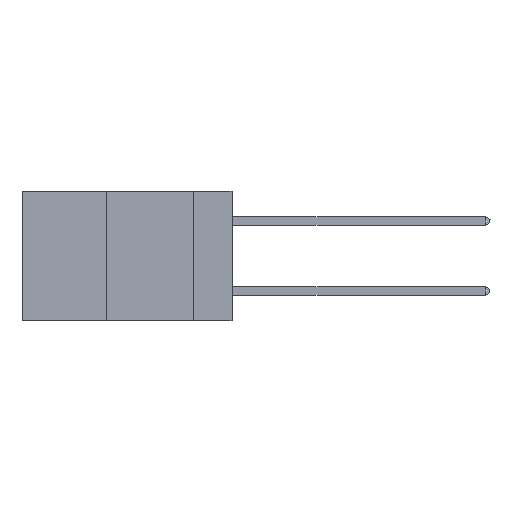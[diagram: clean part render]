
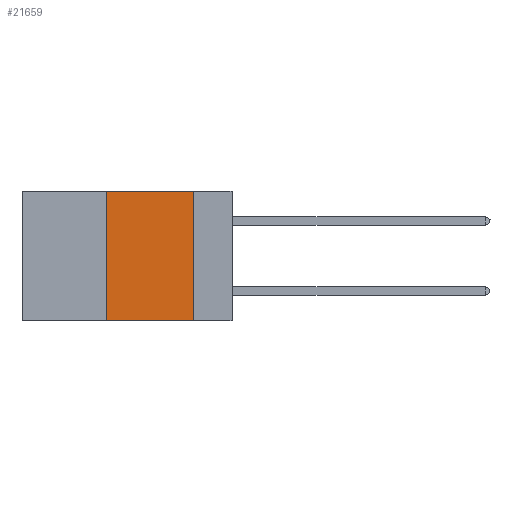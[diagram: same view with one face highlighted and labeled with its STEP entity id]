
A CAD part, left-side view. The second image highlights one B-rep face of the part: STEP entity #21659.
In plain terms, the highlighted planar face has unit normal (-1, 0, 0).
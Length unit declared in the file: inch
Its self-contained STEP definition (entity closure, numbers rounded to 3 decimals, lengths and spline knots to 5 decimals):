
#42 = DIRECTION ( 'NONE',  ( 0., 0., -1. ) ) ;
#2891 = EDGE_CURVE ( 'NONE', #26787, #4432, #26646, .T. ) ;
#3075 = VERTEX_POINT ( 'NONE', #29024 ) ;
#3197 = DIRECTION ( 'NONE',  ( 0., -1., 0. ) ) ;
#4432 = VERTEX_POINT ( 'NONE', #16648 ) ;
#5447 = CARTESIAN_POINT ( 'NONE',  ( 0., 0.36, 0. ) ) ;
#9856 = ORIENTED_EDGE ( 'NONE', *, *, #2891, .F. ) ;
#10792 = DIRECTION ( 'NONE',  ( 0., 0., -1. ) ) ;
#10963 = CARTESIAN_POINT ( 'NONE',  ( 0., 0.6, 0. ) ) ;
#11010 = VERTEX_POINT ( 'NONE', #30320 ) ;
#12275 = LINE ( 'NONE', #31446, #39235 ) ;
#13217 = CARTESIAN_POINT ( 'NONE',  ( 0., 0.6, 0. ) ) ;
#15542 = ORIENTED_EDGE ( 'NONE', *, *, #36780, .T. ) ;
#15550 = CARTESIAN_POINT ( 'NONE',  ( 0., 0.36, 0. ) ) ;
#16310 = FACE_OUTER_BOUND ( 'NONE', #28814, .T. ) ;
#16648 = CARTESIAN_POINT ( 'NONE',  ( 0., 0.11, 0. ) ) ;
#17379 = VECTOR ( 'NONE', #18039, 39.37008 ) ;
#18039 = DIRECTION ( 'NONE',  ( 0., 0., 1. ) ) ;
#19881 = EDGE_CURVE ( 'NONE', #11010, #26787, #33697, .T. ) ;
#20079 = CARTESIAN_POINT ( 'NONE',  ( 0., 0.11, 0. ) ) ;
#21380 = EDGE_CURVE ( 'NONE', #4432, #3075, #29958, .T. ) ;
#21659 = ADVANCED_FACE ( 'NONE', ( #16310 ), #34668, .F. ) ;
#23346 = VECTOR ( 'NONE', #10792, 39.37008 ) ;
#23546 = DIRECTION ( 'NONE',  ( 0., -1., 0. ) ) ;
#26646 = LINE ( 'NONE', #10963, #35731 ) ;
#26787 = VERTEX_POINT ( 'NONE', #15550 ) ;
#27979 = AXIS2_PLACEMENT_3D ( 'NONE', #13217, #31577, #42 ) ;
#28814 = EDGE_LOOP ( 'NONE', ( #30302, #9856, #29311, #15542 ) ) ;
#29024 = CARTESIAN_POINT ( 'NONE',  ( 0., 0.11, -0.37 ) ) ;
#29311 = ORIENTED_EDGE ( 'NONE', *, *, #19881, .F. ) ;
#29958 = LINE ( 'NONE', #20079, #23346 ) ;
#30302 = ORIENTED_EDGE ( 'NONE', *, *, #21380, .F. ) ;
#30320 = CARTESIAN_POINT ( 'NONE',  ( 0., 0.36, -0.37 ) ) ;
#31446 = CARTESIAN_POINT ( 'NONE',  ( 0., 0.6, -0.37 ) ) ;
#31577 = DIRECTION ( 'NONE',  ( 1., 0., 0. ) ) ;
#33697 = LINE ( 'NONE', #5447, #17379 ) ;
#34668 = PLANE ( 'NONE',  #27979 ) ;
#35731 = VECTOR ( 'NONE', #23546, 39.37008 ) ;
#36780 = EDGE_CURVE ( 'NONE', #11010, #3075, #12275, .T. ) ;
#39235 = VECTOR ( 'NONE', #3197, 39.37008 ) ;
